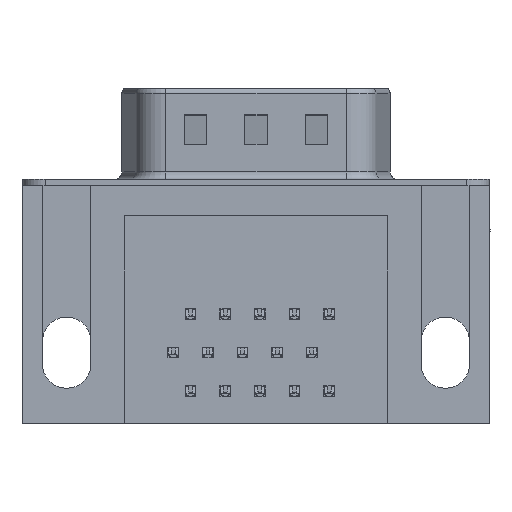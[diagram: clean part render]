
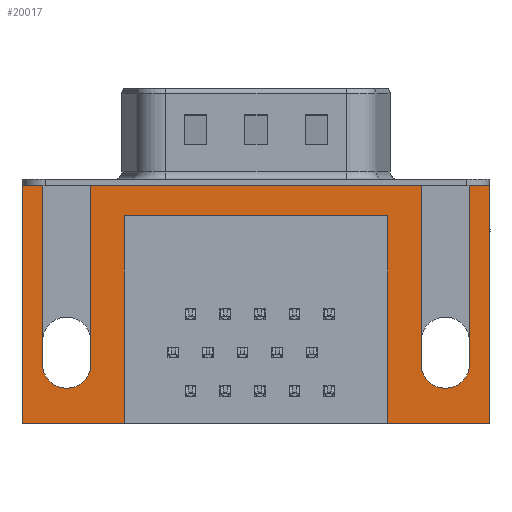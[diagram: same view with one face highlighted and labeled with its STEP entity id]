
A CAD part, front view. The second image highlights one B-rep face of the part: STEP entity #20017.
In plain terms, the highlighted planar face has unit normal (0, -1, 0).
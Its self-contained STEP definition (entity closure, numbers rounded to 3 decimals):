
#201 = ORIENTED_EDGE ( 'NONE', *, *, #9626, .F. ) ;
#254 = EDGE_CURVE ( 'NONE', #21435, #9159, #6636, .T. ) ;
#392 = VECTOR ( 'NONE', #19574, 1000. ) ;
#414 = DIRECTION ( 'NONE',  ( 0., 0., 1. ) ) ;
#636 = ORIENTED_EDGE ( 'NONE', *, *, #5907, .F. ) ;
#654 = ORIENTED_EDGE ( 'NONE', *, *, #254, .F. ) ;
#730 = CARTESIAN_POINT ( 'NONE',  ( -1.6, -6.275, 0. ) ) ;
#889 = VECTOR ( 'NONE', #15719, 1000. ) ;
#891 = ORIENTED_EDGE ( 'NONE', *, *, #2339, .F. ) ;
#1201 = ORIENTED_EDGE ( 'NONE', *, *, #4809, .F. ) ;
#1432 = LINE ( 'NONE', #20511, #889 ) ;
#1436 = AXIS2_PLACEMENT_3D ( 'NONE', #7140, #16055, #414 ) ;
#1517 = AXIS2_PLACEMENT_3D ( 'NONE', #7011, #18528, #8737 ) ;
#1553 = CARTESIAN_POINT ( 'NONE',  ( -2.91, -6.275, -2.5 ) ) ;
#1605 = CARTESIAN_POINT ( 'NONE',  ( 26.59, -6.275, 0. ) ) ;
#1833 = CARTESIAN_POINT ( 'NONE',  ( 21.2, -6.275, -15.7 ) ) ;
#1979 = ORIENTED_EDGE ( 'NONE', *, *, #14726, .F. ) ;
#2068 = VERTEX_POINT ( 'NONE', #7059 ) ;
#2235 = DIRECTION ( 'NONE',  ( -1., 0., 0. ) ) ;
#2263 = VERTEX_POINT ( 'NONE', #10899 ) ;
#2339 = EDGE_CURVE ( 'NONE', #18263, #18349, #21151, .T. ) ;
#3209 = PLANE ( 'NONE',  #14948 ) ;
#3278 = CARTESIAN_POINT ( 'NONE',  ( 1.6, -6.275, -11.78 ) ) ;
#3283 = DIRECTION ( 'NONE',  ( 0., 0., -1. ) ) ;
#3440 = ORIENTED_EDGE ( 'NONE', *, *, #15546, .F. ) ;
#3669 = DIRECTION ( 'NONE',  ( -1., 0., 0. ) ) ;
#3707 = ORIENTED_EDGE ( 'NONE', *, *, #18133, .F. ) ;
#3764 = VECTOR ( 'NONE', #13093, 1000. ) ;
#3991 = VERTEX_POINT ( 'NONE', #18006 ) ;
#4179 = VERTEX_POINT ( 'NONE', #7975 ) ;
#4337 = EDGE_CURVE ( 'NONE', #19334, #2263, #14925, .T. ) ;
#4541 = EDGE_LOOP ( 'NONE', ( #9094, #14355, #654, #1201, #12535, #201, #891, #21509, #13483, #3440, #3707, #16353, #1979, #12538, #13719, #16079, #6384, #636 ) ) ;
#4577 = CARTESIAN_POINT ( 'NONE',  ( 27.9, -6.275, -15.7 ) ) ;
#4809 = EDGE_CURVE ( 'NONE', #11281, #21435, #6085, .T. ) ;
#4862 = VERTEX_POINT ( 'NONE', #8712 ) ;
#5253 = EDGE_CURVE ( 'NONE', #3991, #12302, #7136, .T. ) ;
#5907 = EDGE_CURVE ( 'NONE', #2263, #16255, #1432, .T. ) ;
#6085 = LINE ( 'NONE', #21566, #18718 ) ;
#6110 = VECTOR ( 'NONE', #10049, 1000. ) ;
#6298 = CARTESIAN_POINT ( 'NONE',  ( -2.91, -6.275, -15.7 ) ) ;
#6384 = ORIENTED_EDGE ( 'NONE', *, *, #15274, .T. ) ;
#6420 = CARTESIAN_POINT ( 'NONE',  ( 27.9, -6.275, -15.7 ) ) ;
#6466 = CARTESIAN_POINT ( 'NONE',  ( 0., -6.275, -13.38 ) ) ;
#6508 = CIRCLE ( 'NONE', #1517, 1.6 ) ;
#6545 = CARTESIAN_POINT ( 'NONE',  ( 23.39, -6.275, -11.78 ) ) ;
#6636 = CIRCLE ( 'NONE', #1436, 1.6 ) ;
#6731 = DIRECTION ( 'NONE',  ( 0., 0., 1. ) ) ;
#6767 = DIRECTION ( 'NONE',  ( 0., -1., 0. ) ) ;
#6870 = DIRECTION ( 'NONE',  ( 1., 0., 0. ) ) ;
#7011 = CARTESIAN_POINT ( 'NONE',  ( 24.99, -6.275, -11.78 ) ) ;
#7039 = LINE ( 'NONE', #10236, #15820 ) ;
#7059 = CARTESIAN_POINT ( 'NONE',  ( -1.6, -6.275, -11.78 ) ) ;
#7136 = LINE ( 'NONE', #4577, #19702 ) ;
#7140 = CARTESIAN_POINT ( 'NONE',  ( 24.99, -6.275, -11.78 ) ) ;
#7836 = CARTESIAN_POINT ( 'NONE',  ( 27.9, -6.275, 0. ) ) ;
#7975 = CARTESIAN_POINT ( 'NONE',  ( 3.79, -6.275, -2. ) ) ;
#7980 = AXIS2_PLACEMENT_3D ( 'NONE', #16637, #6767, #18276 ) ;
#8150 = CARTESIAN_POINT ( 'NONE',  ( 3.79, -6.275, -2. ) ) ;
#8351 = LINE ( 'NONE', #6420, #3764 ) ;
#8712 = CARTESIAN_POINT ( 'NONE',  ( 27.9, -6.275, -15.7 ) ) ;
#8737 = DIRECTION ( 'NONE',  ( 0., 0., 1. ) ) ;
#8771 = CARTESIAN_POINT ( 'NONE',  ( 27.9, -6.275, -2.5 ) ) ;
#9065 = LINE ( 'NONE', #8771, #17225 ) ;
#9094 = ORIENTED_EDGE ( 'NONE', *, *, #4337, .F. ) ;
#9098 = CARTESIAN_POINT ( 'NONE',  ( 3.79, -6.275, -2. ) ) ;
#9159 = VERTEX_POINT ( 'NONE', #21258 ) ;
#9320 = VERTEX_POINT ( 'NONE', #1833 ) ;
#9409 = DIRECTION ( 'NONE',  ( 1., 0., 0. ) ) ;
#9449 = CARTESIAN_POINT ( 'NONE',  ( 21.2, -6.275, -2. ) ) ;
#9626 = EDGE_CURVE ( 'NONE', #18349, #14333, #19650, .T. ) ;
#9635 = DIRECTION ( 'NONE',  ( 0., 0., 1. ) ) ;
#10049 = DIRECTION ( 'NONE',  ( 0., 0., 1. ) ) ;
#10236 = CARTESIAN_POINT ( 'NONE',  ( -2.91, -6.275, 0. ) ) ;
#10409 = DIRECTION ( 'NONE',  ( 0., 0., 1. ) ) ;
#10591 = VERTEX_POINT ( 'NONE', #9449 ) ;
#10767 = LINE ( 'NONE', #19405, #12835 ) ;
#10899 = CARTESIAN_POINT ( 'NONE',  ( 26.59, -6.275, 0. ) ) ;
#11107 = CARTESIAN_POINT ( 'NONE',  ( 26.59, -6.275, -11.78 ) ) ;
#11281 = VERTEX_POINT ( 'NONE', #17791 ) ;
#11308 = CARTESIAN_POINT ( 'NONE',  ( -1.6, -6.275, 0. ) ) ;
#11431 = EDGE_CURVE ( 'NONE', #14333, #11281, #7039, .T. ) ;
#11470 = EDGE_CURVE ( 'NONE', #9159, #19334, #6508, .T. ) ;
#11613 = EDGE_CURVE ( 'NONE', #10591, #4179, #16061, .T. ) ;
#11700 = EDGE_CURVE ( 'NONE', #16324, #2068, #18864, .T. ) ;
#11758 = CARTESIAN_POINT ( 'NONE',  ( 21.2, -6.275, -2. ) ) ;
#12280 = VERTEX_POINT ( 'NONE', #17742 ) ;
#12302 = VERTEX_POINT ( 'NONE', #6298 ) ;
#12517 = EDGE_CURVE ( 'NONE', #9320, #10591, #19580, .T. ) ;
#12535 = ORIENTED_EDGE ( 'NONE', *, *, #11431, .F. ) ;
#12538 = ORIENTED_EDGE ( 'NONE', *, *, #11613, .F. ) ;
#12613 = DIRECTION ( 'NONE',  ( 0., 0., -1. ) ) ;
#12835 = VECTOR ( 'NONE', #9635, 1000. ) ;
#13093 = DIRECTION ( 'NONE',  ( -1., 0., 0. ) ) ;
#13308 = CARTESIAN_POINT ( 'NONE',  ( 1.6, -6.275, 0. ) ) ;
#13355 = DIRECTION ( 'NONE',  ( 0., -1., 0. ) ) ;
#13402 = DIRECTION ( 'NONE',  ( 0., 0., 1. ) ) ;
#13483 = ORIENTED_EDGE ( 'NONE', *, *, #11700, .F. ) ;
#13545 = CARTESIAN_POINT ( 'NONE',  ( 1.6, -6.275, 0. ) ) ;
#13659 = VECTOR ( 'NONE', #9409, 1000. ) ;
#13719 = ORIENTED_EDGE ( 'NONE', *, *, #12517, .F. ) ;
#13896 = LINE ( 'NONE', #8150, #392 ) ;
#14333 = VERTEX_POINT ( 'NONE', #13545 ) ;
#14355 = ORIENTED_EDGE ( 'NONE', *, *, #11470, .F. ) ;
#14726 = EDGE_CURVE ( 'NONE', #4179, #3991, #13896, .T. ) ;
#14925 = LINE ( 'NONE', #1605, #6110 ) ;
#14948 = AXIS2_PLACEMENT_3D ( 'NONE', #1553, #13355, #3283 ) ;
#15046 = FACE_OUTER_BOUND ( 'NONE', #4541, .T. ) ;
#15169 = EDGE_CURVE ( 'NONE', #2068, #18263, #15984, .T. ) ;
#15274 = EDGE_CURVE ( 'NONE', #4862, #16255, #9065, .T. ) ;
#15334 = VECTOR ( 'NONE', #6731, 1000. ) ;
#15402 = AXIS2_PLACEMENT_3D ( 'NONE', #17031, #19333, #19309 ) ;
#15546 = EDGE_CURVE ( 'NONE', #12280, #16324, #17476, .T. ) ;
#15689 = DIRECTION ( 'NONE',  ( 0., 0., -1. ) ) ;
#15719 = DIRECTION ( 'NONE',  ( 1., 0., 0. ) ) ;
#15820 = VECTOR ( 'NONE', #6870, 1000. ) ;
#15984 = CIRCLE ( 'NONE', #7980, 1.6 ) ;
#16055 = DIRECTION ( 'NONE',  ( 0., -1., 0. ) ) ;
#16061 = LINE ( 'NONE', #9098, #20831 ) ;
#16079 = ORIENTED_EDGE ( 'NONE', *, *, #20918, .F. ) ;
#16255 = VERTEX_POINT ( 'NONE', #7836 ) ;
#16324 = VERTEX_POINT ( 'NONE', #11308 ) ;
#16353 = ORIENTED_EDGE ( 'NONE', *, *, #5253, .F. ) ;
#16637 = CARTESIAN_POINT ( 'NONE',  ( 0., -6.275, -11.78 ) ) ;
#17031 = CARTESIAN_POINT ( 'NONE',  ( 0., -6.275, -11.78 ) ) ;
#17225 = VECTOR ( 'NONE', #10409, 1000. ) ;
#17476 = LINE ( 'NONE', #19180, #13659 ) ;
#17742 = CARTESIAN_POINT ( 'NONE',  ( -2.91, -6.275, 0. ) ) ;
#17791 = CARTESIAN_POINT ( 'NONE',  ( 23.39, -6.275, 0. ) ) ;
#18006 = CARTESIAN_POINT ( 'NONE',  ( 3.79, -6.275, -15.7 ) ) ;
#18133 = EDGE_CURVE ( 'NONE', #12302, #12280, #10767, .T. ) ;
#18263 = VERTEX_POINT ( 'NONE', #6466 ) ;
#18276 = DIRECTION ( 'NONE',  ( 0., 0., -1. ) ) ;
#18349 = VERTEX_POINT ( 'NONE', #3278 ) ;
#18528 = DIRECTION ( 'NONE',  ( 0., -1., 0. ) ) ;
#18718 = VECTOR ( 'NONE', #15689, 1000. ) ;
#18864 = LINE ( 'NONE', #730, #19364 ) ;
#19180 = CARTESIAN_POINT ( 'NONE',  ( -2.91, -6.275, 0. ) ) ;
#19309 = DIRECTION ( 'NONE',  ( 0., 0., -1. ) ) ;
#19333 = DIRECTION ( 'NONE',  ( 0., -1., 0. ) ) ;
#19334 = VERTEX_POINT ( 'NONE', #11107 ) ;
#19364 = VECTOR ( 'NONE', #12613, 1000. ) ;
#19405 = CARTESIAN_POINT ( 'NONE',  ( -2.91, -6.275, -2.5 ) ) ;
#19574 = DIRECTION ( 'NONE',  ( 0., 0., -1. ) ) ;
#19580 = LINE ( 'NONE', #11758, #20069 ) ;
#19650 = LINE ( 'NONE', #13308, #15334 ) ;
#19702 = VECTOR ( 'NONE', #3669, 1000. ) ;
#20017 = ADVANCED_FACE ( 'NONE', ( #15046 ), #3209, .T. ) ;
#20069 = VECTOR ( 'NONE', #13402, 1000. ) ;
#20511 = CARTESIAN_POINT ( 'NONE',  ( -2.91, -6.275, 0. ) ) ;
#20831 = VECTOR ( 'NONE', #2235, 1000. ) ;
#20918 = EDGE_CURVE ( 'NONE', #4862, #9320, #8351, .T. ) ;
#21151 = CIRCLE ( 'NONE', #15402, 1.6 ) ;
#21258 = CARTESIAN_POINT ( 'NONE',  ( 24.99, -6.275, -13.38 ) ) ;
#21435 = VERTEX_POINT ( 'NONE', #6545 ) ;
#21509 = ORIENTED_EDGE ( 'NONE', *, *, #15169, .F. ) ;
#21566 = CARTESIAN_POINT ( 'NONE',  ( 23.39, -6.275, 0. ) ) ;
